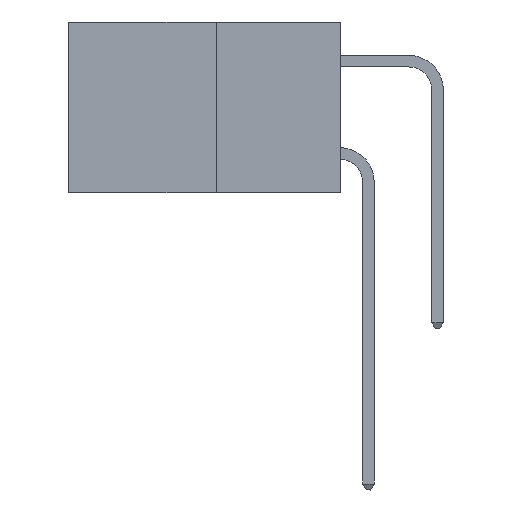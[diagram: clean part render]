
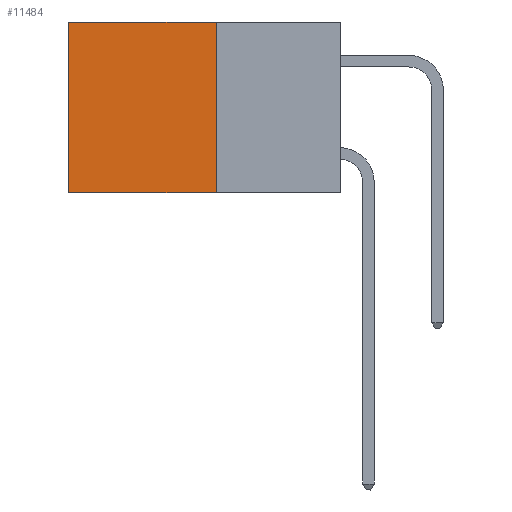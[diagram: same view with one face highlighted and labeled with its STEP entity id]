
A CAD part, left-side view. The second image highlights one B-rep face of the part: STEP entity #11484.
In plain terms, the highlighted planar face has unit normal (-1, 0, 0).
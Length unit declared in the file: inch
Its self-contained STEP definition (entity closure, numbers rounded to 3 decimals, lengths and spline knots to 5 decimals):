
#1386 = DIRECTION ( 'NONE',  ( 0., 0., -1. ) ) ;
#2142 = LINE ( 'NONE', #18835, #27515 ) ;
#2608 = PLANE ( 'NONE',  #20692 ) ;
#3028 = CARTESIAN_POINT ( 'NONE',  ( 0.277, 0.59, -0.37 ) ) ;
#4046 = EDGE_LOOP ( 'NONE', ( #19919, #25242, #29941, #27317 ) ) ;
#5145 = DIRECTION ( 'NONE',  ( 1., 0., 0. ) ) ;
#5575 = DIRECTION ( 'NONE',  ( 0., 0., -1. ) ) ;
#6474 = CARTESIAN_POINT ( 'NONE',  ( 0.277, 0.27, 0. ) ) ;
#7122 = VECTOR ( 'NONE', #26101, 39.37008 ) ;
#9268 = VECTOR ( 'NONE', #27599, 39.37008 ) ;
#9774 = EDGE_CURVE ( 'NONE', #22359, #23789, #2142, .T. ) ;
#10635 = VERTEX_POINT ( 'NONE', #31601 ) ;
#11484 = ADVANCED_FACE ( 'NONE', ( #14293 ), #2608, .F. ) ;
#12086 = LINE ( 'NONE', #3028, #31377 ) ;
#14293 = FACE_OUTER_BOUND ( 'NONE', #4046, .T. ) ;
#15402 = VERTEX_POINT ( 'NONE', #25133 ) ;
#16388 = CARTESIAN_POINT ( 'NONE',  ( 0.277, 0.27, 0. ) ) ;
#17646 = EDGE_CURVE ( 'NONE', #22359, #10635, #20301, .T. ) ;
#18835 = CARTESIAN_POINT ( 'NONE',  ( 0.277, 0.27, -0.37 ) ) ;
#19919 = ORIENTED_EDGE ( 'NONE', *, *, #24032, .T. ) ;
#20024 = CARTESIAN_POINT ( 'NONE',  ( 0.277, 0.27, -0.37 ) ) ;
#20301 = LINE ( 'NONE', #6474, #7122 ) ;
#20692 = AXIS2_PLACEMENT_3D ( 'NONE', #20024, #5145, #22403 ) ;
#22359 = VERTEX_POINT ( 'NONE', #16388 ) ;
#22403 = DIRECTION ( 'NONE',  ( 0., 0., -1. ) ) ;
#23789 = VERTEX_POINT ( 'NONE', #26825 ) ;
#24032 = EDGE_CURVE ( 'NONE', #10635, #15402, #12086, .T. ) ;
#25133 = CARTESIAN_POINT ( 'NONE',  ( 0.277, 0.59, -0.37 ) ) ;
#25187 = CARTESIAN_POINT ( 'NONE',  ( 0.277, 0.27, -0.37 ) ) ;
#25242 = ORIENTED_EDGE ( 'NONE', *, *, #30206, .F. ) ;
#26101 = DIRECTION ( 'NONE',  ( 0., 1., 0. ) ) ;
#26825 = CARTESIAN_POINT ( 'NONE',  ( 0.277, 0.27, -0.37 ) ) ;
#27317 = ORIENTED_EDGE ( 'NONE', *, *, #17646, .T. ) ;
#27515 = VECTOR ( 'NONE', #1386, 39.37008 ) ;
#27599 = DIRECTION ( 'NONE',  ( 0., 1., 0. ) ) ;
#28689 = LINE ( 'NONE', #25187, #9268 ) ;
#29941 = ORIENTED_EDGE ( 'NONE', *, *, #9774, .F. ) ;
#30206 = EDGE_CURVE ( 'NONE', #23789, #15402, #28689, .T. ) ;
#31377 = VECTOR ( 'NONE', #5575, 39.37008 ) ;
#31601 = CARTESIAN_POINT ( 'NONE',  ( 0.277, 0.59, 0. ) ) ;
